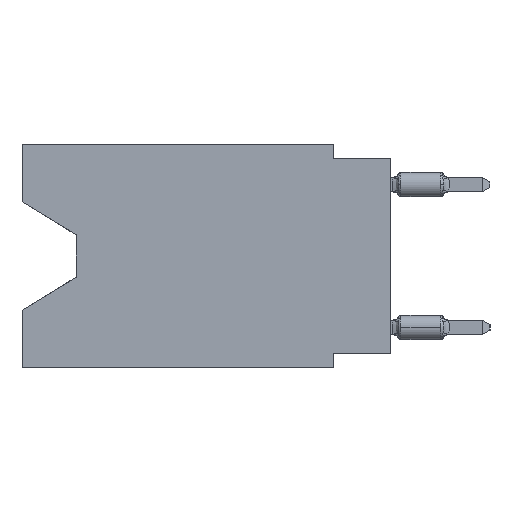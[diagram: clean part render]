
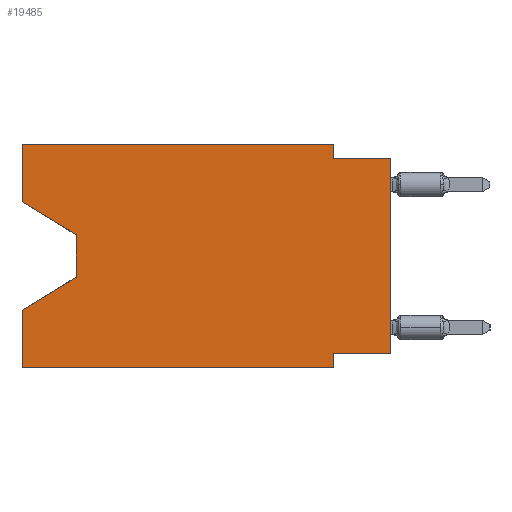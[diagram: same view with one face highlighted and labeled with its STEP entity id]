
A CAD part, left-side view. The second image highlights one B-rep face of the part: STEP entity #19485.
In plain terms, the highlighted planar face has unit normal (-1, 0, 0).
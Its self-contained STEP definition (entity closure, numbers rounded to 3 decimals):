
#472 = CARTESIAN_POINT ( 'NONE',  ( 0., 16.383, 0. ) ) ;
#796 = DIRECTION ( 'NONE',  ( 0., 0., 1. ) ) ;
#856 = VERTEX_POINT ( 'NONE', #19498 ) ;
#1014 = VECTOR ( 'NONE', #9223, 1000. ) ;
#2623 = EDGE_CURVE ( 'NONE', #33746, #9298, #46864, .T. ) ;
#3189 = EDGE_CURVE ( 'NONE', #13007, #51573, #35168, .T. ) ;
#4516 = CARTESIAN_POINT ( 'NONE',  ( 0., 16.383, 0. ) ) ;
#4721 = DIRECTION ( 'NONE',  ( 0., 0., 1. ) ) ;
#5106 = CARTESIAN_POINT ( 'NONE',  ( 0., 16.383, 0. ) ) ;
#5224 = ORIENTED_EDGE ( 'NONE', *, *, #20920, .T. ) ;
#6224 = AXIS2_PLACEMENT_3D ( 'NONE', #27213, #31961, #19022 ) ;
#6583 = CARTESIAN_POINT ( 'NONE',  ( 0., 13.97, -4.013 ) ) ;
#7301 = VERTEX_POINT ( 'NONE', #18209 ) ;
#8446 = CARTESIAN_POINT ( 'NONE',  ( 0., 13.97, -4.013 ) ) ;
#8508 = LINE ( 'NONE', #4516, #28845 ) ;
#9223 = DIRECTION ( 'NONE',  ( 0., -1., 0. ) ) ;
#9294 = VECTOR ( 'NONE', #44592, 1000. ) ;
#9298 = VERTEX_POINT ( 'NONE', #8446 ) ;
#9950 = VERTEX_POINT ( 'NONE', #18570 ) ;
#10013 = CARTESIAN_POINT ( 'NONE',  ( 0., 0., 0. ) ) ;
#10311 = VERTEX_POINT ( 'NONE', #50997 ) ;
#10606 = VERTEX_POINT ( 'NONE', #16627 ) ;
#10689 = DIRECTION ( 'NONE',  ( 0., -0.855, -0.519 ) ) ;
#10783 = VERTEX_POINT ( 'NONE', #19749 ) ;
#10832 = FACE_OUTER_BOUND ( 'NONE', #24754, .T. ) ;
#11390 = VECTOR ( 'NONE', #33560, 1000. ) ;
#12188 = ORIENTED_EDGE ( 'NONE', *, *, #3189, .F. ) ;
#12819 = CARTESIAN_POINT ( 'NONE',  ( 0., 2.54, 0. ) ) ;
#13007 = VERTEX_POINT ( 'NONE', #5106 ) ;
#13037 = DIRECTION ( 'NONE',  ( 0., 0., -1. ) ) ;
#13454 = LINE ( 'NONE', #10013, #16357 ) ;
#13620 = EDGE_CURVE ( 'NONE', #10606, #9950, #36645, .T. ) ;
#14234 = DIRECTION ( 'NONE',  ( 0., 0., 1. ) ) ;
#14641 = ORIENTED_EDGE ( 'NONE', *, *, #48505, .F. ) ;
#15199 = VECTOR ( 'NONE', #17961, 1000. ) ;
#15291 = ORIENTED_EDGE ( 'NONE', *, *, #25825, .T. ) ;
#16357 = VECTOR ( 'NONE', #14234, 1000. ) ;
#16627 = CARTESIAN_POINT ( 'NONE',  ( 0., 13.97, -5.893 ) ) ;
#16743 = CARTESIAN_POINT ( 'NONE',  ( 0., 0., -9.271 ) ) ;
#17030 = EDGE_CURVE ( 'NONE', #51573, #10311, #47971, .T. ) ;
#17961 = DIRECTION ( 'NONE',  ( 0., -1., 0. ) ) ;
#17997 = VERTEX_POINT ( 'NONE', #49418 ) ;
#18209 = CARTESIAN_POINT ( 'NONE',  ( 0., 16.383, -9.906 ) ) ;
#18570 = CARTESIAN_POINT ( 'NONE',  ( 0., 16.383, -7.36 ) ) ;
#18807 = EDGE_CURVE ( 'NONE', #856, #35030, #37346, .T. ) ;
#19022 = DIRECTION ( 'NONE',  ( 0., 0., -1. ) ) ;
#19029 = ORIENTED_EDGE ( 'NONE', *, *, #17030, .F. ) ;
#19485 = ADVANCED_FACE ( 'NONE', ( #10832 ), #52018, .F. ) ;
#19498 = CARTESIAN_POINT ( 'NONE',  ( 0., 0., -9.271 ) ) ;
#19749 = CARTESIAN_POINT ( 'NONE',  ( 0., 2.54, -9.906 ) ) ;
#20425 = CARTESIAN_POINT ( 'NONE',  ( 0., 16.383, -2.546 ) ) ;
#20920 = EDGE_CURVE ( 'NONE', #9298, #10606, #25636, .T. ) ;
#24228 = DIRECTION ( 'NONE',  ( 0., 0.855, -0.519 ) ) ;
#24658 = LINE ( 'NONE', #36013, #41738 ) ;
#24754 = EDGE_LOOP ( 'NONE', ( #49788, #5224, #42097, #14641, #39208, #50820, #26710, #15291, #43600, #19029, #12188, #36500 ) ) ;
#24761 = EDGE_CURVE ( 'NONE', #7301, #10783, #26387, .T. ) ;
#25636 = LINE ( 'NONE', #6583, #11390 ) ;
#25825 = EDGE_CURVE ( 'NONE', #856, #17997, #13454, .T. ) ;
#26387 = LINE ( 'NONE', #49884, #1014 ) ;
#26710 = ORIENTED_EDGE ( 'NONE', *, *, #18807, .F. ) ;
#27213 = CARTESIAN_POINT ( 'NONE',  ( 0., 16.383, 0. ) ) ;
#28431 = DIRECTION ( 'NONE',  ( 0., 0., -1. ) ) ;
#28445 = CARTESIAN_POINT ( 'NONE',  ( 0., 13.97, -5.893 ) ) ;
#28845 = VECTOR ( 'NONE', #796, 1000. ) ;
#29858 = LINE ( 'NONE', #37519, #15199 ) ;
#31961 = DIRECTION ( 'NONE',  ( 1., 0., 0. ) ) ;
#33560 = DIRECTION ( 'NONE',  ( 0., 0., -1. ) ) ;
#33746 = VERTEX_POINT ( 'NONE', #20425 ) ;
#34876 = VECTOR ( 'NONE', #37612, 1000. ) ;
#35003 = EDGE_CURVE ( 'NONE', #35030, #10783, #24658, .T. ) ;
#35030 = VERTEX_POINT ( 'NONE', #48937 ) ;
#35168 = LINE ( 'NONE', #472, #9294 ) ;
#35400 = VECTOR ( 'NONE', #4721, 1000. ) ;
#36013 = CARTESIAN_POINT ( 'NONE',  ( 0., 2.54, -9.906 ) ) ;
#36500 = ORIENTED_EDGE ( 'NONE', *, *, #43583, .F. ) ;
#36645 = LINE ( 'NONE', #28445, #43045 ) ;
#37346 = LINE ( 'NONE', #16743, #34876 ) ;
#37519 = CARTESIAN_POINT ( 'NONE',  ( 0., 0., -0.635 ) ) ;
#37612 = DIRECTION ( 'NONE',  ( 0., 1., 0. ) ) ;
#37726 = CARTESIAN_POINT ( 'NONE',  ( 0., 16.383, 0. ) ) ;
#38437 = CARTESIAN_POINT ( 'NONE',  ( 0., 16.383, -2.546 ) ) ;
#39068 = VECTOR ( 'NONE', #28431, 1000. ) ;
#39208 = ORIENTED_EDGE ( 'NONE', *, *, #24761, .T. ) ;
#39904 = EDGE_CURVE ( 'NONE', #10311, #17997, #29858, .T. ) ;
#40472 = VECTOR ( 'NONE', #10689, 1000. ) ;
#41738 = VECTOR ( 'NONE', #13037, 1000. ) ;
#42097 = ORIENTED_EDGE ( 'NONE', *, *, #13620, .T. ) ;
#43045 = VECTOR ( 'NONE', #24228, 1000. ) ;
#43583 = EDGE_CURVE ( 'NONE', #33746, #13007, #8508, .T. ) ;
#43600 = ORIENTED_EDGE ( 'NONE', *, *, #39904, .F. ) ;
#44592 = DIRECTION ( 'NONE',  ( 0., -1., 0. ) ) ;
#45655 = LINE ( 'NONE', #37726, #35400 ) ;
#46864 = LINE ( 'NONE', #38437, #40472 ) ;
#47971 = LINE ( 'NONE', #48515, #39068 ) ;
#48505 = EDGE_CURVE ( 'NONE', #7301, #9950, #45655, .T. ) ;
#48515 = CARTESIAN_POINT ( 'NONE',  ( 0., 2.54, 0. ) ) ;
#48937 = CARTESIAN_POINT ( 'NONE',  ( 0., 2.54, -9.271 ) ) ;
#49418 = CARTESIAN_POINT ( 'NONE',  ( 0., 0., -0.635 ) ) ;
#49788 = ORIENTED_EDGE ( 'NONE', *, *, #2623, .T. ) ;
#49884 = CARTESIAN_POINT ( 'NONE',  ( 0., 16.383, -9.906 ) ) ;
#50820 = ORIENTED_EDGE ( 'NONE', *, *, #35003, .F. ) ;
#50997 = CARTESIAN_POINT ( 'NONE',  ( 0., 2.54, -0.635 ) ) ;
#51573 = VERTEX_POINT ( 'NONE', #12819 ) ;
#52018 = PLANE ( 'NONE',  #6224 ) ;
